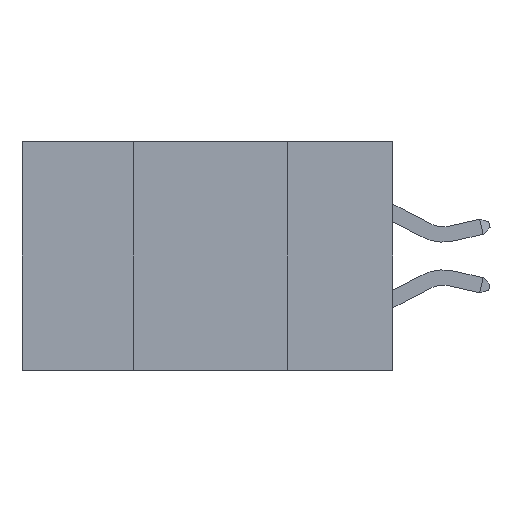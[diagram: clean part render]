
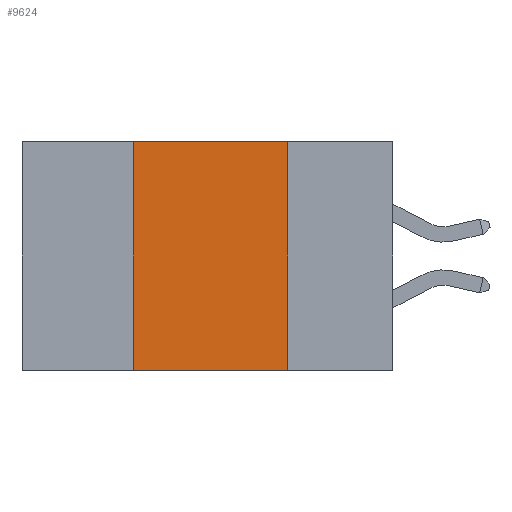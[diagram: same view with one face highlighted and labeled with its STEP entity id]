
A CAD part, left-side view. The second image highlights one B-rep face of the part: STEP entity #9624.
In plain terms, the highlighted planar face has unit normal (-1, 0, 0).
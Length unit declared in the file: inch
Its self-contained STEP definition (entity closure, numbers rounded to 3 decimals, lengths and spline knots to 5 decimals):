
#124 = DIRECTION ( 'NONE',  ( 0., -1., 0. ) ) ;
#784 = LINE ( 'NONE', #2017, #4890 ) ;
#1065 = CARTESIAN_POINT ( 'NONE',  ( 0., 0.6, 0. ) ) ;
#2017 = CARTESIAN_POINT ( 'NONE',  ( 0., 0.42, 0. ) ) ;
#2290 = CARTESIAN_POINT ( 'NONE',  ( 0., 0.6, -0.37 ) ) ;
#2704 = ORIENTED_EDGE ( 'NONE', *, *, #4986, .F. ) ;
#3162 = DIRECTION ( 'NONE',  ( 0., 0., 1. ) ) ;
#3257 = CARTESIAN_POINT ( 'NONE',  ( 0., 0.42, -0.37 ) ) ;
#3365 = DIRECTION ( 'NONE',  ( 0., 0., -1. ) ) ;
#3440 = EDGE_CURVE ( 'NONE', #9139, #9605, #784, .T. ) ;
#3608 = VECTOR ( 'NONE', #9294, 39.37008 ) ;
#3735 = ORIENTED_EDGE ( 'NONE', *, *, #8984, .F. ) ;
#3762 = LINE ( 'NONE', #5992, #3608 ) ;
#4377 = VERTEX_POINT ( 'NONE', #4521 ) ;
#4443 = DIRECTION ( 'NONE',  ( 1., 0., 0. ) ) ;
#4521 = CARTESIAN_POINT ( 'NONE',  ( 0., 0.17, -0.37 ) ) ;
#4650 = CARTESIAN_POINT ( 'NONE',  ( 0., 0.42, 0. ) ) ;
#4890 = VECTOR ( 'NONE', #3162, 39.37008 ) ;
#4986 = EDGE_CURVE ( 'NONE', #8732, #4377, #5934, .T. ) ;
#5443 = LINE ( 'NONE', #2290, #6627 ) ;
#5934 = LINE ( 'NONE', #7944, #9553 ) ;
#5992 = CARTESIAN_POINT ( 'NONE',  ( 0., 0.6, 0. ) ) ;
#6627 = VECTOR ( 'NONE', #124, 39.37008 ) ;
#6681 = ORIENTED_EDGE ( 'NONE', *, *, #3440, .F. ) ;
#7280 = CARTESIAN_POINT ( 'NONE',  ( 0., 0.17, 0. ) ) ;
#7810 = PLANE ( 'NONE',  #12353 ) ;
#7944 = CARTESIAN_POINT ( 'NONE',  ( 0., 0.17, 0. ) ) ;
#8602 = EDGE_LOOP ( 'NONE', ( #2704, #3735, #6681, #11284 ) ) ;
#8732 = VERTEX_POINT ( 'NONE', #7280 ) ;
#8893 = FACE_OUTER_BOUND ( 'NONE', #8602, .T. ) ;
#8984 = EDGE_CURVE ( 'NONE', #9605, #8732, #3762, .T. ) ;
#9139 = VERTEX_POINT ( 'NONE', #3257 ) ;
#9294 = DIRECTION ( 'NONE',  ( 0., -1., 0. ) ) ;
#9553 = VECTOR ( 'NONE', #10112, 39.37008 ) ;
#9605 = VERTEX_POINT ( 'NONE', #4650 ) ;
#9624 = ADVANCED_FACE ( 'NONE', ( #8893 ), #7810, .F. ) ;
#10112 = DIRECTION ( 'NONE',  ( 0., 0., -1. ) ) ;
#11284 = ORIENTED_EDGE ( 'NONE', *, *, #12505, .T. ) ;
#12353 = AXIS2_PLACEMENT_3D ( 'NONE', #1065, #4443, #3365 ) ;
#12505 = EDGE_CURVE ( 'NONE', #9139, #4377, #5443, .T. ) ;
